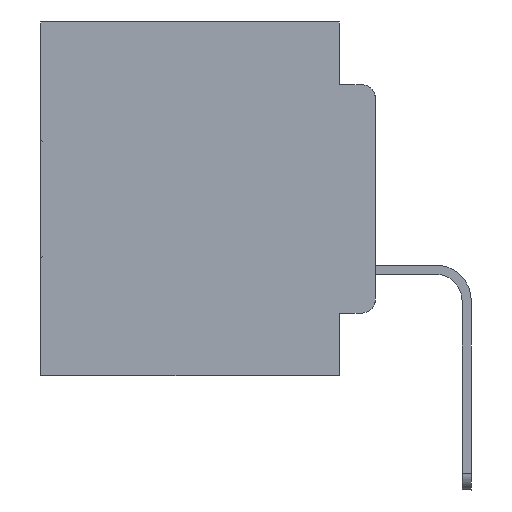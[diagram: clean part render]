
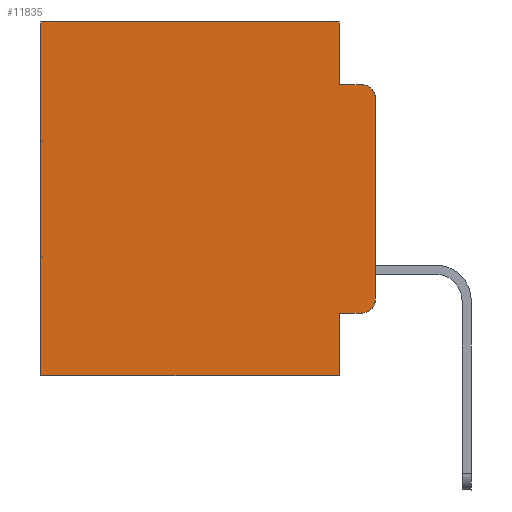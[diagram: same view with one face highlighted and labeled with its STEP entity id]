
A CAD part, left-side view. The second image highlights one B-rep face of the part: STEP entity #11835.
In plain terms, the highlighted planar face has unit normal (-1, 0, 0).
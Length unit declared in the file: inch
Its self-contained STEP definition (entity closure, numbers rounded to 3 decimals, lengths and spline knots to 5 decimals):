
#182 = DIRECTION ( 'NONE',  ( -1., 0., 0. ) ) ;
#451 = VERTEX_POINT ( 'NONE', #3299 ) ;
#643 = CARTESIAN_POINT ( 'NONE',  ( 0.298, 0.473, 0. ) ) ;
#725 = CARTESIAN_POINT ( 'NONE',  ( 0.298, 0.051, -0.0885 ) ) ;
#1244 = VECTOR ( 'NONE', #2239, 39.37008 ) ;
#2239 = DIRECTION ( 'NONE',  ( 0., 0., -1. ) ) ;
#2341 = CARTESIAN_POINT ( 'NONE',  ( 0.298, 0.473, 0. ) ) ;
#2362 = EDGE_CURVE ( 'NONE', #15448, #18337, #11885, .T. ) ;
#2583 = DIRECTION ( 'NONE',  ( -1., 0., 0. ) ) ;
#2959 = VERTEX_POINT ( 'NONE', #8904 ) ;
#3299 = CARTESIAN_POINT ( 'NONE',  ( 0.298, 0.02, -0.0885 ) ) ;
#3334 = VECTOR ( 'NONE', #25389, 39.37008 ) ;
#4067 = VECTOR ( 'NONE', #16057, 39.37008 ) ;
#4558 = EDGE_LOOP ( 'NONE', ( #9417, #23864, #10887, #30251, #27178, #14491, #28063, #15244, #16384, #25098 ) ) ;
#6836 = CARTESIAN_POINT ( 'NONE',  ( 0.298, 0.02, -0.4115 ) ) ;
#7169 = DIRECTION ( 'NONE',  ( 0., 0., -1. ) ) ;
#7283 = CARTESIAN_POINT ( 'NONE',  ( 0.298, 0.02, -0.3915 ) ) ;
#7701 = LINE ( 'NONE', #26306, #1244 ) ;
#7818 = EDGE_CURVE ( 'NONE', #20487, #451, #31142, .T. ) ;
#8003 = VERTEX_POINT ( 'NONE', #22339 ) ;
#8575 = FACE_OUTER_BOUND ( 'NONE', #4558, .T. ) ;
#8608 = LINE ( 'NONE', #23552, #4067 ) ;
#8732 = EDGE_CURVE ( 'NONE', #8848, #19316, #29171, .T. ) ;
#8848 = VERTEX_POINT ( 'NONE', #9706 ) ;
#8904 = CARTESIAN_POINT ( 'NONE',  ( 0.298, 0., -0.3915 ) ) ;
#8924 = AXIS2_PLACEMENT_3D ( 'NONE', #7283, #182, #7169 ) ;
#9417 = ORIENTED_EDGE ( 'NONE', *, *, #16736, .F. ) ;
#9442 = CARTESIAN_POINT ( 'NONE',  ( 0.298, 0., 0. ) ) ;
#9480 = DIRECTION ( 'NONE',  ( 0., -1., 0. ) ) ;
#9706 = CARTESIAN_POINT ( 'NONE',  ( 0.298, 0.051, -0.4115 ) ) ;
#9838 = VECTOR ( 'NONE', #26293, 39.37008 ) ;
#10344 = VECTOR ( 'NONE', #15674, 39.37008 ) ;
#10576 = LINE ( 'NONE', #16758, #9838 ) ;
#10887 = ORIENTED_EDGE ( 'NONE', *, *, #18560, .F. ) ;
#11791 = CARTESIAN_POINT ( 'NONE',  ( 0.298, 0., 0. ) ) ;
#11835 = ADVANCED_FACE ( 'NONE', ( #8575 ), #31189, .F. ) ;
#11885 = LINE ( 'NONE', #9442, #15286 ) ;
#11957 = EDGE_CURVE ( 'NONE', #18337, #8003, #28690, .T. ) ;
#12369 = CIRCLE ( 'NONE', #8924, 0.02 ) ;
#14316 = DIRECTION ( 'NONE',  ( 0., 1., 0. ) ) ;
#14491 = ORIENTED_EDGE ( 'NONE', *, *, #11957, .T. ) ;
#14775 = DIRECTION ( 'NONE',  ( 0., 0., -1. ) ) ;
#15244 = ORIENTED_EDGE ( 'NONE', *, *, #16463, .F. ) ;
#15286 = VECTOR ( 'NONE', #14316, 39.37008 ) ;
#15448 = VERTEX_POINT ( 'NONE', #15534 ) ;
#15534 = CARTESIAN_POINT ( 'NONE',  ( 0.298, 0.051, 0. ) ) ;
#15674 = DIRECTION ( 'NONE',  ( 0., 0., -1. ) ) ;
#16057 = DIRECTION ( 'NONE',  ( 0., 1., 0. ) ) ;
#16251 = VERTEX_POINT ( 'NONE', #30765 ) ;
#16384 = ORIENTED_EDGE ( 'NONE', *, *, #8732, .T. ) ;
#16463 = EDGE_CURVE ( 'NONE', #8848, #16251, #10576, .T. ) ;
#16540 = VECTOR ( 'NONE', #21607, 39.37008 ) ;
#16736 = EDGE_CURVE ( 'NONE', #20487, #2959, #26365, .T. ) ;
#16758 = CARTESIAN_POINT ( 'NONE',  ( 0.298, 0.051, 0. ) ) ;
#17405 = CARTESIAN_POINT ( 'NONE',  ( 0.298, 0.02, -0.1085 ) ) ;
#18337 = VERTEX_POINT ( 'NONE', #2341 ) ;
#18560 = EDGE_CURVE ( 'NONE', #28644, #451, #20784, .T. ) ;
#19316 = VERTEX_POINT ( 'NONE', #6836 ) ;
#19356 = EDGE_CURVE ( 'NONE', #16251, #8003, #8608, .T. ) ;
#20487 = VERTEX_POINT ( 'NONE', #23169 ) ;
#20784 = LINE ( 'NONE', #725, #3334 ) ;
#21485 = EDGE_CURVE ( 'NONE', #15448, #28644, #7701, .T. ) ;
#21607 = DIRECTION ( 'NONE',  ( 0., 0., -1. ) ) ;
#22339 = CARTESIAN_POINT ( 'NONE',  ( 0.298, 0.473, -0.5 ) ) ;
#23169 = CARTESIAN_POINT ( 'NONE',  ( 0.298, 0., -0.1085 ) ) ;
#23552 = CARTESIAN_POINT ( 'NONE',  ( 0.298, 0., -0.5 ) ) ;
#23864 = ORIENTED_EDGE ( 'NONE', *, *, #7818, .T. ) ;
#24302 = AXIS2_PLACEMENT_3D ( 'NONE', #17405, #2583, #14775 ) ;
#24466 = EDGE_CURVE ( 'NONE', #19316, #2959, #12369, .T. ) ;
#25098 = ORIENTED_EDGE ( 'NONE', *, *, #24466, .T. ) ;
#25389 = DIRECTION ( 'NONE',  ( 0., -1., 0. ) ) ;
#25421 = AXIS2_PLACEMENT_3D ( 'NONE', #11791, #28744, #31295 ) ;
#26293 = DIRECTION ( 'NONE',  ( 0., 0., -1. ) ) ;
#26306 = CARTESIAN_POINT ( 'NONE',  ( 0.298, 0.051, 0. ) ) ;
#26365 = LINE ( 'NONE', #30618, #10344 ) ;
#27178 = ORIENTED_EDGE ( 'NONE', *, *, #2362, .T. ) ;
#27343 = CARTESIAN_POINT ( 'NONE',  ( 0.298, 0.051, -0.0885 ) ) ;
#28031 = VECTOR ( 'NONE', #9480, 39.37008 ) ;
#28063 = ORIENTED_EDGE ( 'NONE', *, *, #19356, .F. ) ;
#28644 = VERTEX_POINT ( 'NONE', #27343 ) ;
#28690 = LINE ( 'NONE', #643, #16540 ) ;
#28744 = DIRECTION ( 'NONE',  ( 1., 0., 0. ) ) ;
#29097 = CARTESIAN_POINT ( 'NONE',  ( 0.298, 0.051, -0.4115 ) ) ;
#29171 = LINE ( 'NONE', #29097, #28031 ) ;
#30251 = ORIENTED_EDGE ( 'NONE', *, *, #21485, .F. ) ;
#30618 = CARTESIAN_POINT ( 'NONE',  ( 0.298, 0., 0. ) ) ;
#30765 = CARTESIAN_POINT ( 'NONE',  ( 0.298, 0.051, -0.5 ) ) ;
#31142 = CIRCLE ( 'NONE', #24302, 0.02 ) ;
#31189 = PLANE ( 'NONE',  #25421 ) ;
#31295 = DIRECTION ( 'NONE',  ( 0., 0., -1. ) ) ;
